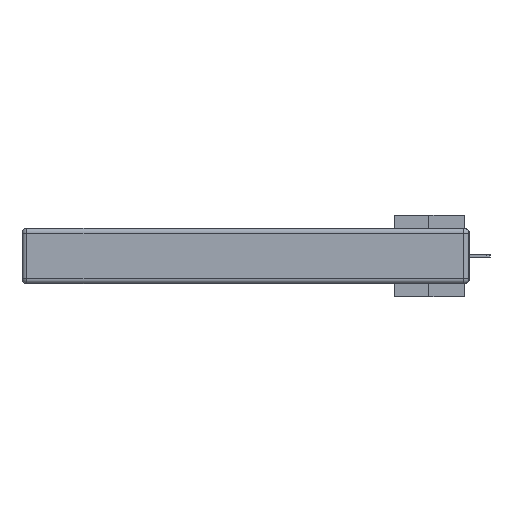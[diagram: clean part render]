
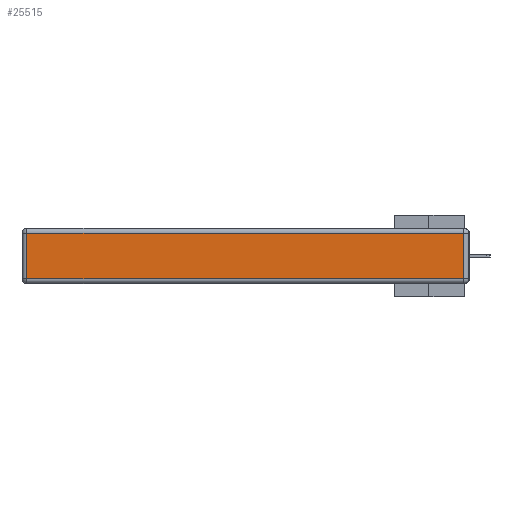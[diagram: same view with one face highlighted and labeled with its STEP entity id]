
A CAD part, left-side view. The second image highlights one B-rep face of the part: STEP entity #25515.
In plain terms, the highlighted planar face has unit normal (-1, 0, 0).
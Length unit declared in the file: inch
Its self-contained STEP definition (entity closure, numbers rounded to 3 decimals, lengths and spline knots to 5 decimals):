
#1496 = ORIENTED_EDGE ( 'NONE', *, *, #35699, .T. ) ;
#2279 = DIRECTION ( 'NONE',  ( 0., 0., 1. ) ) ;
#3529 = VERTEX_POINT ( 'NONE', #23446 ) ;
#3828 = DIRECTION ( 'NONE',  ( -1., 0., 0. ) ) ;
#5107 = VECTOR ( 'NONE', #32675, 39.37008 ) ;
#5683 = CARTESIAN_POINT ( 'NONE',  ( 0., 2.72, -0.313 ) ) ;
#8121 = LINE ( 'NONE', #31654, #8219 ) ;
#8219 = VECTOR ( 'NONE', #11364, 39.37008 ) ;
#9760 = LINE ( 'NONE', #19509, #5107 ) ;
#11364 = DIRECTION ( 'NONE',  ( 0., 0., -1. ) ) ;
#12203 = LINE ( 'NONE', #38549, #19397 ) ;
#16053 = ORIENTED_EDGE ( 'NONE', *, *, #19797, .T. ) ;
#16374 = EDGE_LOOP ( 'NONE', ( #30007, #1496, #16053, #18695 ) ) ;
#18695 = ORIENTED_EDGE ( 'NONE', *, *, #32443, .T. ) ;
#19218 = LINE ( 'NONE', #25704, #28741 ) ;
#19397 = VECTOR ( 'NONE', #2279, 39.37008 ) ;
#19509 = CARTESIAN_POINT ( 'NONE',  ( 0., 0., -0.313 ) ) ;
#19797 = EDGE_CURVE ( 'NONE', #22951, #30677, #19218, .T. ) ;
#22951 = VERTEX_POINT ( 'NONE', #35141 ) ;
#23446 = CARTESIAN_POINT ( 'NONE',  ( 0., 0.03, -0.313 ) ) ;
#24180 = CARTESIAN_POINT ( 'NONE',  ( 0., 2.72, -0.03 ) ) ;
#25515 = ADVANCED_FACE ( 'NONE', ( #27674 ), #28891, .T. ) ;
#25704 = CARTESIAN_POINT ( 'NONE',  ( 0., 2.75, -0.03 ) ) ;
#26504 = AXIS2_PLACEMENT_3D ( 'NONE', #42074, #3828, #39251 ) ;
#27674 = FACE_OUTER_BOUND ( 'NONE', #16374, .T. ) ;
#28741 = VECTOR ( 'NONE', #38877, 39.37008 ) ;
#28891 = PLANE ( 'NONE',  #26504 ) ;
#30007 = ORIENTED_EDGE ( 'NONE', *, *, #41933, .T. ) ;
#30677 = VERTEX_POINT ( 'NONE', #24180 ) ;
#31654 = CARTESIAN_POINT ( 'NONE',  ( 0., 2.72, -0.343 ) ) ;
#32443 = EDGE_CURVE ( 'NONE', #30677, #36163, #8121, .T. ) ;
#32675 = DIRECTION ( 'NONE',  ( 0., -1., 0. ) ) ;
#35141 = CARTESIAN_POINT ( 'NONE',  ( 0., 0.03, -0.03 ) ) ;
#35699 = EDGE_CURVE ( 'NONE', #3529, #22951, #12203, .T. ) ;
#36163 = VERTEX_POINT ( 'NONE', #5683 ) ;
#38549 = CARTESIAN_POINT ( 'NONE',  ( 0., 0.03, -0.343 ) ) ;
#38877 = DIRECTION ( 'NONE',  ( 0., 1., 0. ) ) ;
#39251 = DIRECTION ( 'NONE',  ( 0., 0., 1. ) ) ;
#41933 = EDGE_CURVE ( 'NONE', #36163, #3529, #9760, .T. ) ;
#42074 = CARTESIAN_POINT ( 'NONE',  ( 0., 0., -0.343 ) ) ;
